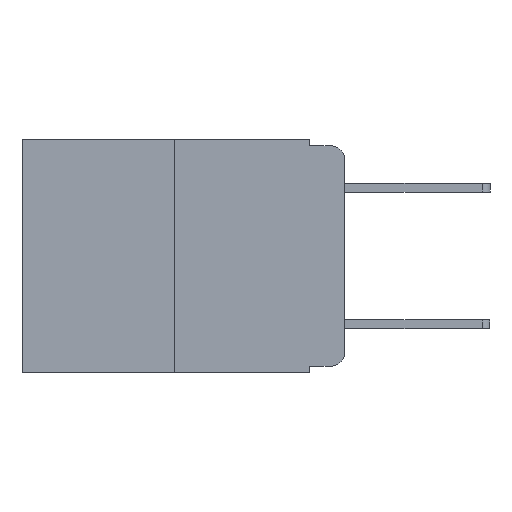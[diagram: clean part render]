
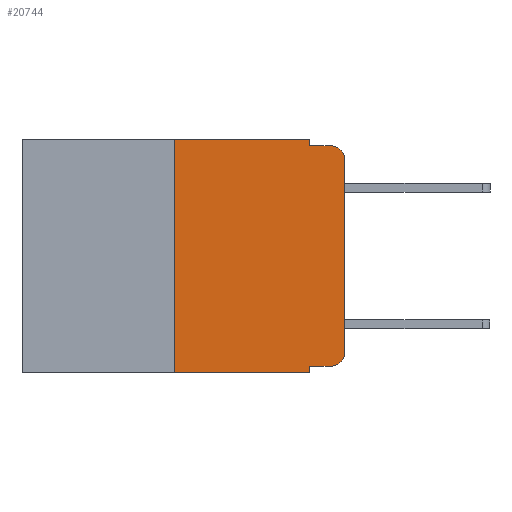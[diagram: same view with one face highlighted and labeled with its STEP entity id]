
A CAD part, left-side view. The second image highlights one B-rep face of the part: STEP entity #20744.
In plain terms, the highlighted planar face has unit normal (-1, 0, 0).
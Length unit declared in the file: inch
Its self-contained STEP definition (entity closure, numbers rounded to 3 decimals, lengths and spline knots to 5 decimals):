
#172 = LINE ( 'NONE', #20447, #15716 ) ;
#392 = AXIS2_PLACEMENT_3D ( 'NONE', #15394, #3288, #17396 ) ;
#632 = CARTESIAN_POINT ( 'NONE',  ( 0., 0.051, -0.333 ) ) ;
#899 = DIRECTION ( 'NONE',  ( 0., -1., 0. ) ) ;
#926 = ORIENTED_EDGE ( 'NONE', *, *, #2498, .T. ) ;
#1095 = VERTEX_POINT ( 'NONE', #14159 ) ;
#1790 = VERTEX_POINT ( 'NONE', #5596 ) ;
#2304 = ORIENTED_EDGE ( 'NONE', *, *, #15038, .F. ) ;
#2498 = EDGE_CURVE ( 'NONE', #10135, #1095, #8550, .T. ) ;
#3007 = CARTESIAN_POINT ( 'NONE',  ( 0., 0.051, 0. ) ) ;
#3106 = CARTESIAN_POINT ( 'NONE',  ( 0., 0.25, -0.343 ) ) ;
#3161 = VECTOR ( 'NONE', #17470, 39.37008 ) ;
#3288 = DIRECTION ( 'NONE',  ( -1., 0., 0. ) ) ;
#3356 = ORIENTED_EDGE ( 'NONE', *, *, #23754, .F. ) ;
#3820 = EDGE_LOOP ( 'NONE', ( #11639, #25211, #25566, #3356, #3981, #2304, #12284, #22841, #926, #18075 ) ) ;
#3981 = ORIENTED_EDGE ( 'NONE', *, *, #15751, .F. ) ;
#4347 = VERTEX_POINT ( 'NONE', #20469 ) ;
#4731 = VECTOR ( 'NONE', #8125, 39.37008 ) ;
#5160 = PLANE ( 'NONE',  #6858 ) ;
#5434 = LINE ( 'NONE', #7089, #10198 ) ;
#5596 = CARTESIAN_POINT ( 'NONE',  ( 0., 0.051, -0.343 ) ) ;
#5965 = CARTESIAN_POINT ( 'NONE',  ( 0., 0.051, 0. ) ) ;
#6034 = VERTEX_POINT ( 'NONE', #21905 ) ;
#6091 = CARTESIAN_POINT ( 'NONE',  ( 0., 0.25, 0. ) ) ;
#6435 = DIRECTION ( 'NONE',  ( 0., -1., 0. ) ) ;
#6762 = EDGE_CURVE ( 'NONE', #9795, #16675, #21995, .T. ) ;
#6858 = AXIS2_PLACEMENT_3D ( 'NONE', #13220, #23100, #11297 ) ;
#7071 = EDGE_CURVE ( 'NONE', #1095, #6034, #15234, .T. ) ;
#7089 = CARTESIAN_POINT ( 'NONE',  ( 0., 0., 0. ) ) ;
#8125 = DIRECTION ( 'NONE',  ( 0., 0., 1. ) ) ;
#8247 = DIRECTION ( 'NONE',  ( -1., 0., 0. ) ) ;
#8550 = LINE ( 'NONE', #11401, #3161 ) ;
#8619 = CARTESIAN_POINT ( 'NONE',  ( 0., 0.051, 0. ) ) ;
#8630 = EDGE_CURVE ( 'NONE', #6034, #9795, #5434, .T. ) ;
#8688 = LINE ( 'NONE', #20834, #13468 ) ;
#9795 = VERTEX_POINT ( 'NONE', #11800 ) ;
#10135 = VERTEX_POINT ( 'NONE', #632 ) ;
#10136 = LINE ( 'NONE', #6091, #4731 ) ;
#10198 = VECTOR ( 'NONE', #22999, 39.37008 ) ;
#10341 = VECTOR ( 'NONE', #25790, 39.37008 ) ;
#11297 = DIRECTION ( 'NONE',  ( 0., 0., -1. ) ) ;
#11401 = CARTESIAN_POINT ( 'NONE',  ( 0., 0.051, -0.333 ) ) ;
#11639 = ORIENTED_EDGE ( 'NONE', *, *, #8630, .T. ) ;
#11800 = CARTESIAN_POINT ( 'NONE',  ( 0., 0., -0.03 ) ) ;
#12284 = ORIENTED_EDGE ( 'NONE', *, *, #24833, .T. ) ;
#13220 = CARTESIAN_POINT ( 'NONE',  ( 0., 0.473, 0. ) ) ;
#13468 = VECTOR ( 'NONE', #899, 39.37008 ) ;
#13497 = CARTESIAN_POINT ( 'NONE',  ( 0., 0.02, -0.01 ) ) ;
#14159 = CARTESIAN_POINT ( 'NONE',  ( 0., 0.02, -0.333 ) ) ;
#15038 = EDGE_CURVE ( 'NONE', #19535, #4347, #10136, .T. ) ;
#15234 = CIRCLE ( 'NONE', #18009, 0.02 ) ;
#15382 = EDGE_CURVE ( 'NONE', #15760, #16675, #18525, .T. ) ;
#15394 = CARTESIAN_POINT ( 'NONE',  ( 0., 0.02, -0.03 ) ) ;
#15716 = VECTOR ( 'NONE', #6435, 39.37008 ) ;
#15751 = EDGE_CURVE ( 'NONE', #4347, #20537, #172, .T. ) ;
#15760 = VERTEX_POINT ( 'NONE', #16570 ) ;
#16570 = CARTESIAN_POINT ( 'NONE',  ( 0., 0.051, -0.01 ) ) ;
#16675 = VERTEX_POINT ( 'NONE', #13497 ) ;
#17396 = DIRECTION ( 'NONE',  ( 0., 0., -1. ) ) ;
#17470 = DIRECTION ( 'NONE',  ( 0., -1., 0. ) ) ;
#18009 = AXIS2_PLACEMENT_3D ( 'NONE', #20206, #8247, #22137 ) ;
#18075 = ORIENTED_EDGE ( 'NONE', *, *, #7071, .T. ) ;
#18139 = LINE ( 'NONE', #5965, #10341 ) ;
#18525 = LINE ( 'NONE', #23172, #23096 ) ;
#19350 = LINE ( 'NONE', #3007, #23904 ) ;
#19535 = VERTEX_POINT ( 'NONE', #3106 ) ;
#20206 = CARTESIAN_POINT ( 'NONE',  ( 0., 0.02, -0.313 ) ) ;
#20447 = CARTESIAN_POINT ( 'NONE',  ( 0., 0.473, 0. ) ) ;
#20469 = CARTESIAN_POINT ( 'NONE',  ( 0., 0.25, 0. ) ) ;
#20537 = VERTEX_POINT ( 'NONE', #8619 ) ;
#20744 = ADVANCED_FACE ( 'NONE', ( #21666 ), #5160, .F. ) ;
#20834 = CARTESIAN_POINT ( 'NONE',  ( 0., 0.473, -0.343 ) ) ;
#21304 = DIRECTION ( 'NONE',  ( 0., -1., 0. ) ) ;
#21666 = FACE_OUTER_BOUND ( 'NONE', #3820, .T. ) ;
#21905 = CARTESIAN_POINT ( 'NONE',  ( 0., 0., -0.313 ) ) ;
#21995 = CIRCLE ( 'NONE', #392, 0.02 ) ;
#22137 = DIRECTION ( 'NONE',  ( 0., 0., -1. ) ) ;
#22841 = ORIENTED_EDGE ( 'NONE', *, *, #23417, .F. ) ;
#22909 = DIRECTION ( 'NONE',  ( 0., 0., -1. ) ) ;
#22999 = DIRECTION ( 'NONE',  ( 0., 0., 1. ) ) ;
#23096 = VECTOR ( 'NONE', #21304, 39.37008 ) ;
#23100 = DIRECTION ( 'NONE',  ( 1., 0., 0. ) ) ;
#23172 = CARTESIAN_POINT ( 'NONE',  ( 0., 0.051, -0.01 ) ) ;
#23417 = EDGE_CURVE ( 'NONE', #10135, #1790, #18139, .T. ) ;
#23754 = EDGE_CURVE ( 'NONE', #20537, #15760, #19350, .T. ) ;
#23904 = VECTOR ( 'NONE', #22909, 39.37008 ) ;
#24833 = EDGE_CURVE ( 'NONE', #19535, #1790, #8688, .T. ) ;
#25211 = ORIENTED_EDGE ( 'NONE', *, *, #6762, .T. ) ;
#25566 = ORIENTED_EDGE ( 'NONE', *, *, #15382, .F. ) ;
#25790 = DIRECTION ( 'NONE',  ( 0., 0., -1. ) ) ;
